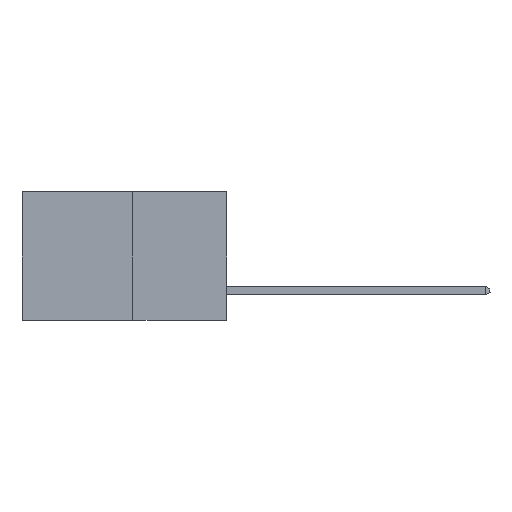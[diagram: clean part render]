
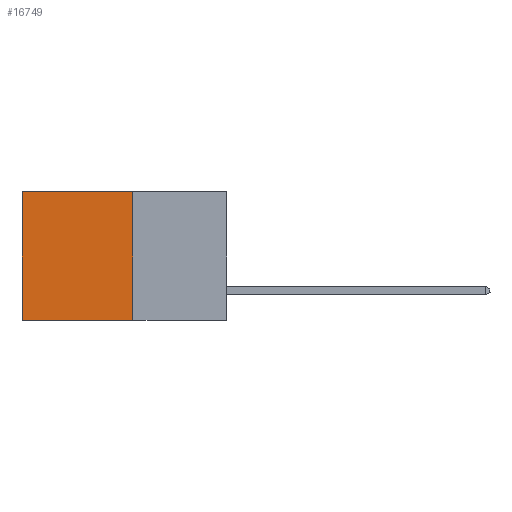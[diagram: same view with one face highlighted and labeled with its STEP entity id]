
A CAD part, left-side view. The second image highlights one B-rep face of the part: STEP entity #16749.
In plain terms, the highlighted planar face has unit normal (-1, 0, 0).
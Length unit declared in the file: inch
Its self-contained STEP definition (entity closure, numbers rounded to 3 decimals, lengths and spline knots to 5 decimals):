
#1931 = CARTESIAN_POINT ( 'NONE',  ( 0.277, 0.59, -0.37 ) ) ;
#2885 = ORIENTED_EDGE ( 'NONE', *, *, #27659, .T. ) ;
#3237 = ORIENTED_EDGE ( 'NONE', *, *, #17054, .F. ) ;
#3484 = DIRECTION ( 'NONE',  ( 0., 0., -1. ) ) ;
#4115 = VECTOR ( 'NONE', #18968, 39.37008 ) ;
#4819 = LINE ( 'NONE', #25576, #4115 ) ;
#6867 = VERTEX_POINT ( 'NONE', #9693 ) ;
#6898 = DIRECTION ( 'NONE',  ( 0., 1., 0. ) ) ;
#9693 = CARTESIAN_POINT ( 'NONE',  ( 0.277, 0.27, 0. ) ) ;
#10151 = VERTEX_POINT ( 'NONE', #18557 ) ;
#12090 = CARTESIAN_POINT ( 'NONE',  ( 0.277, 0.27, -0.37 ) ) ;
#12112 = LINE ( 'NONE', #1931, #24670 ) ;
#12286 = VERTEX_POINT ( 'NONE', #23724 ) ;
#12595 = FACE_OUTER_BOUND ( 'NONE', #24828, .T. ) ;
#13425 = PLANE ( 'NONE',  #22128 ) ;
#15706 = DIRECTION ( 'NONE',  ( 0., 0., -1. ) ) ;
#16749 = ADVANCED_FACE ( 'NONE', ( #12595 ), #13425, .F. ) ;
#17049 = CARTESIAN_POINT ( 'NONE',  ( 0.277, 0.59, 0. ) ) ;
#17054 = EDGE_CURVE ( 'NONE', #10151, #12286, #4819, .T. ) ;
#17903 = CARTESIAN_POINT ( 'NONE',  ( 0.277, 0.27, -0.37 ) ) ;
#18115 = ORIENTED_EDGE ( 'NONE', *, *, #22220, .F. ) ;
#18135 = CARTESIAN_POINT ( 'NONE',  ( 0.277, 0.27, 0. ) ) ;
#18557 = CARTESIAN_POINT ( 'NONE',  ( 0.277, 0.27, -0.37 ) ) ;
#18968 = DIRECTION ( 'NONE',  ( 0., 1., 0. ) ) ;
#19620 = VERTEX_POINT ( 'NONE', #17049 ) ;
#20036 = DIRECTION ( 'NONE',  ( 0., 0., -1. ) ) ;
#21116 = LINE ( 'NONE', #18135, #26929 ) ;
#22128 = AXIS2_PLACEMENT_3D ( 'NONE', #17903, #28925, #15706 ) ;
#22220 = EDGE_CURVE ( 'NONE', #6867, #10151, #23115, .T. ) ;
#22575 = ORIENTED_EDGE ( 'NONE', *, *, #24931, .T. ) ;
#23115 = LINE ( 'NONE', #12090, #27540 ) ;
#23724 = CARTESIAN_POINT ( 'NONE',  ( 0.277, 0.59, -0.37 ) ) ;
#24670 = VECTOR ( 'NONE', #20036, 39.37008 ) ;
#24828 = EDGE_LOOP ( 'NONE', ( #22575, #3237, #18115, #2885 ) ) ;
#24931 = EDGE_CURVE ( 'NONE', #19620, #12286, #12112, .T. ) ;
#25576 = CARTESIAN_POINT ( 'NONE',  ( 0.277, 0.27, -0.37 ) ) ;
#26929 = VECTOR ( 'NONE', #6898, 39.37008 ) ;
#27540 = VECTOR ( 'NONE', #3484, 39.37008 ) ;
#27659 = EDGE_CURVE ( 'NONE', #6867, #19620, #21116, .T. ) ;
#28925 = DIRECTION ( 'NONE',  ( 1., 0., 0. ) ) ;
